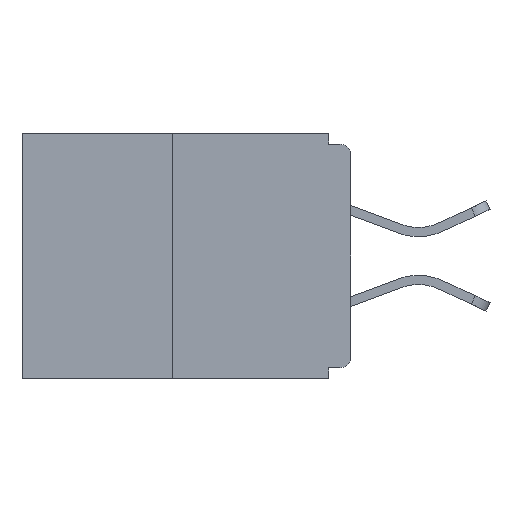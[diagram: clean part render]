
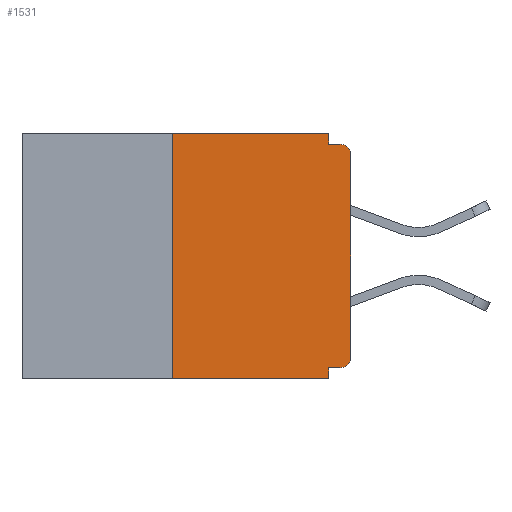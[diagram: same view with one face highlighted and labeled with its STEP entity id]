
A CAD part, left-side view. The second image highlights one B-rep face of the part: STEP entity #1531.
In plain terms, the highlighted planar face has unit normal (-1, 0, 0).
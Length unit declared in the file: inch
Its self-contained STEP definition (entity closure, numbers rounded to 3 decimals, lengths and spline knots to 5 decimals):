
#128 = DIRECTION ( 'NONE',  ( 1., 0., 0. ) ) ;
#190 = ORIENTED_EDGE ( 'NONE', *, *, #8772, .T. ) ;
#248 = CARTESIAN_POINT ( 'NONE',  ( 0., 0.015, -0.03 ) ) ;
#778 = CARTESIAN_POINT ( 'NONE',  ( 0., 0.031, -0.328 ) ) ;
#877 = ORIENTED_EDGE ( 'NONE', *, *, #9524, .F. ) ;
#1067 = PLANE ( 'NONE',  #1146 ) ;
#1114 = DIRECTION ( 'NONE',  ( -1., 0., 0. ) ) ;
#1146 = AXIS2_PLACEMENT_3D ( 'NONE', #4912, #128, #5856 ) ;
#1196 = EDGE_CURVE ( 'NONE', #3802, #5758, #1978, .T. ) ;
#1271 = VERTEX_POINT ( 'NONE', #4937 ) ;
#1531 = ADVANCED_FACE ( 'NONE', ( #7648 ), #1067, .F. ) ;
#1766 = VERTEX_POINT ( 'NONE', #8201 ) ;
#1978 = LINE ( 'NONE', #2039, #3119 ) ;
#2039 = CARTESIAN_POINT ( 'NONE',  ( 0., 0.031, 0. ) ) ;
#2062 = CARTESIAN_POINT ( 'NONE',  ( 0., 0.015, -0.313 ) ) ;
#2137 = CARTESIAN_POINT ( 'NONE',  ( 0., 0.031, -0.343 ) ) ;
#2490 = LINE ( 'NONE', #9002, #4786 ) ;
#2574 = VECTOR ( 'NONE', #4795, 39.37008 ) ;
#2585 = EDGE_CURVE ( 'NONE', #4710, #9829, #3478, .T. ) ;
#2783 = CARTESIAN_POINT ( 'NONE',  ( 0., 0.25, 0. ) ) ;
#2929 = AXIS2_PLACEMENT_3D ( 'NONE', #2062, #1114, #9657 ) ;
#3051 = LINE ( 'NONE', #7868, #5988 ) ;
#3066 = EDGE_LOOP ( 'NONE', ( #10555, #5923, #12434, #4278, #6322, #190, #5862, #6324, #877, #8435 ) ) ;
#3119 = VECTOR ( 'NONE', #11831, 39.37008 ) ;
#3478 = LINE ( 'NONE', #11958, #10894 ) ;
#3796 = DIRECTION ( 'NONE',  ( -1., 0., 0. ) ) ;
#3802 = VERTEX_POINT ( 'NONE', #8094 ) ;
#4278 = ORIENTED_EDGE ( 'NONE', *, *, #8309, .F. ) ;
#4710 = VERTEX_POINT ( 'NONE', #8010 ) ;
#4735 = CIRCLE ( 'NONE', #2929, 0.015 ) ;
#4786 = VECTOR ( 'NONE', #8058, 39.37008 ) ;
#4795 = DIRECTION ( 'NONE',  ( 0., 0., -1. ) ) ;
#4826 = DIRECTION ( 'NONE',  ( 0., -1., 0. ) ) ;
#4843 = CARTESIAN_POINT ( 'NONE',  ( 0., 0.031, -0.015 ) ) ;
#4912 = CARTESIAN_POINT ( 'NONE',  ( 0., 0.46, 0. ) ) ;
#4937 = CARTESIAN_POINT ( 'NONE',  ( 0., 0.015, -0.328 ) ) ;
#5286 = EDGE_CURVE ( 'NONE', #10778, #8122, #9707, .T. ) ;
#5758 = VERTEX_POINT ( 'NONE', #4843 ) ;
#5828 = LINE ( 'NONE', #7688, #7066 ) ;
#5856 = DIRECTION ( 'NONE',  ( 0., 0., -1. ) ) ;
#5862 = ORIENTED_EDGE ( 'NONE', *, *, #10624, .T. ) ;
#5884 = EDGE_CURVE ( 'NONE', #1271, #11143, #2490, .T. ) ;
#5923 = ORIENTED_EDGE ( 'NONE', *, *, #2585, .F. ) ;
#5988 = VECTOR ( 'NONE', #4826, 39.37008 ) ;
#6070 = CARTESIAN_POINT ( 'NONE',  ( 0., 0., -0.015 ) ) ;
#6158 = EDGE_CURVE ( 'NONE', #9829, #3802, #3051, .T. ) ;
#6322 = ORIENTED_EDGE ( 'NONE', *, *, #5884, .F. ) ;
#6324 = ORIENTED_EDGE ( 'NONE', *, *, #5286, .T. ) ;
#6797 = EDGE_CURVE ( 'NONE', #4710, #1766, #9161, .T. ) ;
#7021 = DIRECTION ( 'NONE',  ( 0., -1., 0. ) ) ;
#7038 = CARTESIAN_POINT ( 'NONE',  ( 0., 0., -0.03 ) ) ;
#7066 = VECTOR ( 'NONE', #8498, 39.37008 ) ;
#7220 = DIRECTION ( 'NONE',  ( 0., 0., 1. ) ) ;
#7648 = FACE_OUTER_BOUND ( 'NONE', #3066, .T. ) ;
#7661 = DIRECTION ( 'NONE',  ( 0., 0., -1. ) ) ;
#7688 = CARTESIAN_POINT ( 'NONE',  ( 0., 0., 0. ) ) ;
#7866 = DIRECTION ( 'NONE',  ( 0., -1., 0. ) ) ;
#7868 = CARTESIAN_POINT ( 'NONE',  ( 0., 0.46, 0. ) ) ;
#8010 = CARTESIAN_POINT ( 'NONE',  ( 0., 0.25, -0.343 ) ) ;
#8058 = DIRECTION ( 'NONE',  ( 0., 1., 0. ) ) ;
#8094 = CARTESIAN_POINT ( 'NONE',  ( 0., 0.031, 0. ) ) ;
#8122 = VERTEX_POINT ( 'NONE', #9291 ) ;
#8201 = CARTESIAN_POINT ( 'NONE',  ( 0., 0.031, -0.343 ) ) ;
#8309 = EDGE_CURVE ( 'NONE', #11143, #1766, #11747, .T. ) ;
#8435 = ORIENTED_EDGE ( 'NONE', *, *, #1196, .F. ) ;
#8498 = DIRECTION ( 'NONE',  ( 0., 0., 1. ) ) ;
#8772 = EDGE_CURVE ( 'NONE', #1271, #9126, #4735, .T. ) ;
#8997 = VECTOR ( 'NONE', #7866, 39.37008 ) ;
#9002 = CARTESIAN_POINT ( 'NONE',  ( 0., 0., -0.328 ) ) ;
#9126 = VERTEX_POINT ( 'NONE', #10460 ) ;
#9161 = LINE ( 'NONE', #11820, #11663 ) ;
#9291 = CARTESIAN_POINT ( 'NONE',  ( 0., 0.015, -0.015 ) ) ;
#9524 = EDGE_CURVE ( 'NONE', #5758, #8122, #9756, .T. ) ;
#9657 = DIRECTION ( 'NONE',  ( 0., 0., -1. ) ) ;
#9707 = CIRCLE ( 'NONE', #10302, 0.015 ) ;
#9756 = LINE ( 'NONE', #6070, #8997 ) ;
#9829 = VERTEX_POINT ( 'NONE', #2783 ) ;
#10302 = AXIS2_PLACEMENT_3D ( 'NONE', #248, #3796, #7661 ) ;
#10460 = CARTESIAN_POINT ( 'NONE',  ( 0., 0., -0.313 ) ) ;
#10555 = ORIENTED_EDGE ( 'NONE', *, *, #6158, .F. ) ;
#10624 = EDGE_CURVE ( 'NONE', #9126, #10778, #5828, .T. ) ;
#10778 = VERTEX_POINT ( 'NONE', #7038 ) ;
#10894 = VECTOR ( 'NONE', #7220, 39.37008 ) ;
#11143 = VERTEX_POINT ( 'NONE', #778 ) ;
#11663 = VECTOR ( 'NONE', #7021, 39.37008 ) ;
#11747 = LINE ( 'NONE', #2137, #2574 ) ;
#11820 = CARTESIAN_POINT ( 'NONE',  ( 0., 0.46, -0.343 ) ) ;
#11831 = DIRECTION ( 'NONE',  ( 0., 0., -1. ) ) ;
#11958 = CARTESIAN_POINT ( 'NONE',  ( 0., 0.25, 0. ) ) ;
#12434 = ORIENTED_EDGE ( 'NONE', *, *, #6797, .T. ) ;
